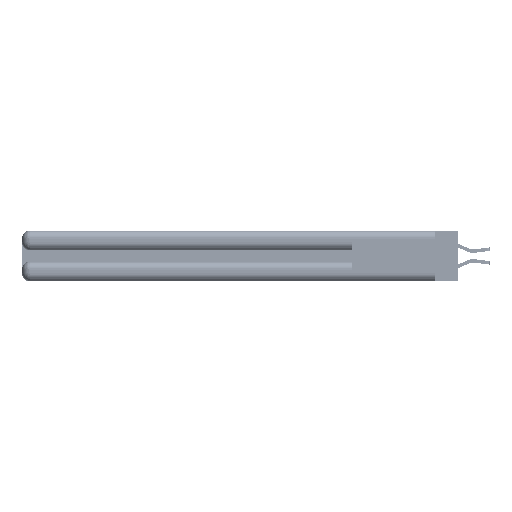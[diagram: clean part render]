
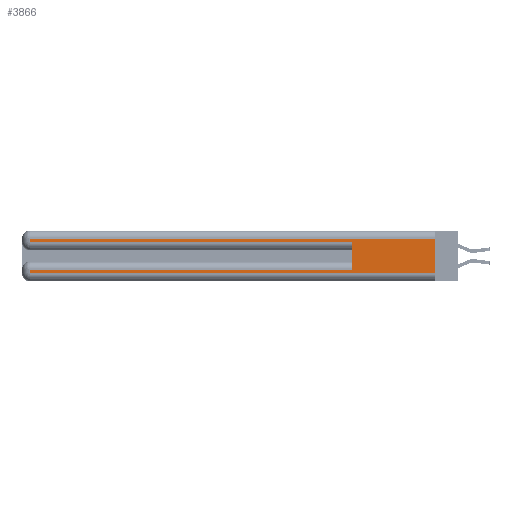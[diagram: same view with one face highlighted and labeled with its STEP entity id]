
A CAD part, left-side view. The second image highlights one B-rep face of the part: STEP entity #3866.
In plain terms, the highlighted planar face has unit normal (-1, 0, 0).
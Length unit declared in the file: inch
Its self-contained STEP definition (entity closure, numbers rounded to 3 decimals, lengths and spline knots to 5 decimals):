
#594 = CARTESIAN_POINT ( 'NONE',  ( 0., 2.94, 0.37 ) ) ;
#645 = ORIENTED_EDGE ( 'NONE', *, *, #5161, .T. ) ;
#2105 = LINE ( 'NONE', #39683, #13554 ) ;
#2538 = CARTESIAN_POINT ( 'NONE',  ( 0., 0., 0.37 ) ) ;
#3407 = VERTEX_POINT ( 'NONE', #23086 ) ;
#3866 = ADVANCED_FACE ( 'NONE', ( #5296 ), #13991, .F. ) ;
#4216 = VERTEX_POINT ( 'NONE', #31050 ) ;
#4234 = ORIENTED_EDGE ( 'NONE', *, *, #9755, .T. ) ;
#5161 = EDGE_CURVE ( 'NONE', #16363, #37943, #48325, .T. ) ;
#5296 = FACE_OUTER_BOUND ( 'NONE', #11996, .T. ) ;
#6437 = DIRECTION ( 'NONE',  ( 0., 0., -1. ) ) ;
#8831 = DIRECTION ( 'NONE',  ( 0., 0., 1. ) ) ;
#9755 = EDGE_CURVE ( 'NONE', #47978, #3407, #22496, .T. ) ;
#11514 = ORIENTED_EDGE ( 'NONE', *, *, #37199, .T. ) ;
#11996 = EDGE_LOOP ( 'NONE', ( #40087, #45513, #4234, #26469, #30063, #645, #11514, #12699 ) ) ;
#12699 = ORIENTED_EDGE ( 'NONE', *, *, #40725, .T. ) ;
#13108 = VECTOR ( 'NONE', #17724, 39.37008 ) ;
#13554 = VECTOR ( 'NONE', #16703, 39.37008 ) ;
#13991 = PLANE ( 'NONE',  #48999 ) ;
#14522 = EDGE_CURVE ( 'NONE', #4216, #47978, #42514, .T. ) ;
#14582 = VERTEX_POINT ( 'NONE', #33300 ) ;
#14839 = LINE ( 'NONE', #25822, #45408 ) ;
#16106 = EDGE_CURVE ( 'NONE', #4216, #28789, #2105, .T. ) ;
#16363 = VERTEX_POINT ( 'NONE', #48835 ) ;
#16553 = VECTOR ( 'NONE', #17494, 39.37008 ) ;
#16703 = DIRECTION ( 'NONE',  ( 0., 0., -1. ) ) ;
#17494 = DIRECTION ( 'NONE',  ( 0., 1., 0. ) ) ;
#17724 = DIRECTION ( 'NONE',  ( 0., 1., 0. ) ) ;
#18659 = LINE ( 'NONE', #21865, #40239 ) ;
#19520 = CARTESIAN_POINT ( 'NONE',  ( 0., 0., 0.06 ) ) ;
#19920 = LINE ( 'NONE', #31010, #28931 ) ;
#21865 = CARTESIAN_POINT ( 'NONE',  ( 0., 0., 0.285 ) ) ;
#22496 = LINE ( 'NONE', #594, #38392 ) ;
#23086 = CARTESIAN_POINT ( 'NONE',  ( 0., 2.94, 0.285 ) ) ;
#23114 = VECTOR ( 'NONE', #8831, 39.37008 ) ;
#25710 = DIRECTION ( 'NONE',  ( 0., -1., 0. ) ) ;
#25822 = CARTESIAN_POINT ( 'NONE',  ( 0., 2.94, 0.37 ) ) ;
#26469 = ORIENTED_EDGE ( 'NONE', *, *, #32802, .T. ) ;
#28789 = VERTEX_POINT ( 'NONE', #19520 ) ;
#28931 = VECTOR ( 'NONE', #42589, 39.37008 ) ;
#29385 = DIRECTION ( 'NONE',  ( 1., 0., 0. ) ) ;
#29682 = DIRECTION ( 'NONE',  ( 0., 0., -1. ) ) ;
#30063 = ORIENTED_EDGE ( 'NONE', *, *, #30199, .F. ) ;
#30199 = EDGE_CURVE ( 'NONE', #16363, #46795, #45899, .T. ) ;
#31010 = CARTESIAN_POINT ( 'NONE',  ( 0., 0., 0.06 ) ) ;
#31050 = CARTESIAN_POINT ( 'NONE',  ( 0., 0., 0.31 ) ) ;
#31301 = DIRECTION ( 'NONE',  ( 0., 0., -1. ) ) ;
#31783 = CARTESIAN_POINT ( 'NONE',  ( 0., 0.6, 0.145 ) ) ;
#32765 = CARTESIAN_POINT ( 'NONE',  ( 0., 0., 0.085 ) ) ;
#32802 = EDGE_CURVE ( 'NONE', #3407, #46795, #18659, .T. ) ;
#33300 = CARTESIAN_POINT ( 'NONE',  ( 0., 2.94, 0.06 ) ) ;
#33414 = CARTESIAN_POINT ( 'NONE',  ( 0., 2.94, 0.31 ) ) ;
#35285 = CARTESIAN_POINT ( 'NONE',  ( 0., 2.94, 0.085 ) ) ;
#37199 = EDGE_CURVE ( 'NONE', #37943, #14582, #14839, .T. ) ;
#37943 = VERTEX_POINT ( 'NONE', #35285 ) ;
#38392 = VECTOR ( 'NONE', #31301, 39.37008 ) ;
#39683 = CARTESIAN_POINT ( 'NONE',  ( 0., 0., 0.37 ) ) ;
#40087 = ORIENTED_EDGE ( 'NONE', *, *, #16106, .F. ) ;
#40239 = VECTOR ( 'NONE', #25710, 39.37008 ) ;
#40687 = CARTESIAN_POINT ( 'NONE',  ( 0., 0., 0.31 ) ) ;
#40725 = EDGE_CURVE ( 'NONE', #14582, #28789, #19920, .T. ) ;
#41771 = CARTESIAN_POINT ( 'NONE',  ( 0., 0.6, 0.285 ) ) ;
#42514 = LINE ( 'NONE', #40687, #13108 ) ;
#42589 = DIRECTION ( 'NONE',  ( 0., -1., 0. ) ) ;
#45408 = VECTOR ( 'NONE', #29682, 39.37008 ) ;
#45513 = ORIENTED_EDGE ( 'NONE', *, *, #14522, .T. ) ;
#45899 = LINE ( 'NONE', #31783, #23114 ) ;
#46795 = VERTEX_POINT ( 'NONE', #41771 ) ;
#47978 = VERTEX_POINT ( 'NONE', #33414 ) ;
#48325 = LINE ( 'NONE', #32765, #16553 ) ;
#48835 = CARTESIAN_POINT ( 'NONE',  ( 0., 0.6, 0.085 ) ) ;
#48999 = AXIS2_PLACEMENT_3D ( 'NONE', #2538, #29385, #6437 ) ;
